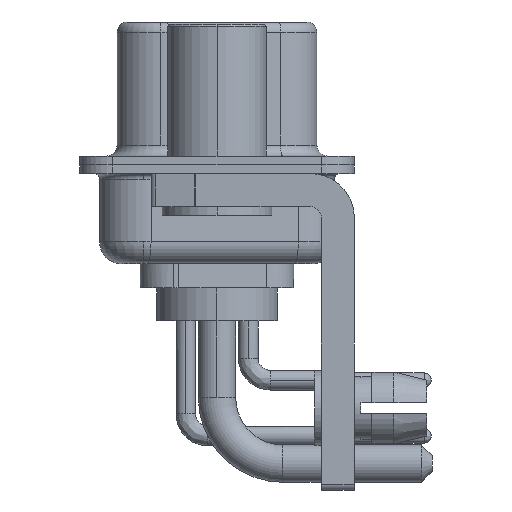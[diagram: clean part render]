
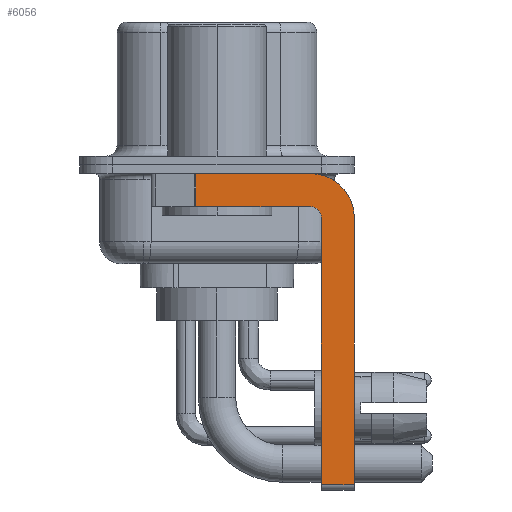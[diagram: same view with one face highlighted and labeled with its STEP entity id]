
A CAD part, left-side view. The second image highlights one B-rep face of the part: STEP entity #6056.
In plain terms, the highlighted planar face has unit normal (-1, 0, 0).
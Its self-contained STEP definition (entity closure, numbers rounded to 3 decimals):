
#176 = DIRECTION ( 'NONE',  ( 0., 0., -1. ) ) ;
#267 = CARTESIAN_POINT ( 'NONE',  ( -2.9, -4.75, -14.55 ) ) ;
#996 = DIRECTION ( 'NONE',  ( 0., 0., -1. ) ) ;
#1007 = AXIS2_PLACEMENT_3D ( 'NONE', #15987, #13909, #996 ) ;
#1122 = CARTESIAN_POINT ( 'NONE',  ( -2.9, -4.25, -2.4 ) ) ;
#1993 = VECTOR ( 'NONE', #10875, 1000. ) ;
#2012 = CARTESIAN_POINT ( 'NONE',  ( -2.9, -6.25, -14.55 ) ) ;
#2116 = ORIENTED_EDGE ( 'NONE', *, *, #15926, .F. ) ;
#2143 = CARTESIAN_POINT ( 'NONE',  ( -2.9, -4.75, -2.4 ) ) ;
#2294 = LINE ( 'NONE', #19380, #18590 ) ;
#2717 = CARTESIAN_POINT ( 'NONE',  ( -2.9, 0.978, -0.4 ) ) ;
#3073 = LINE ( 'NONE', #21999, #12347 ) ;
#3507 = CIRCLE ( 'NONE', #4383, 0.5 ) ;
#3719 = ORIENTED_EDGE ( 'NONE', *, *, #20674, .F. ) ;
#4383 = AXIS2_PLACEMENT_3D ( 'NONE', #13957, #26971, #12120 ) ;
#5748 = LINE ( 'NONE', #22566, #7154 ) ;
#6056 = ADVANCED_FACE ( 'NONE', ( #15854 ), #16405, .F. ) ;
#6746 = ORIENTED_EDGE ( 'NONE', *, *, #23729, .T. ) ;
#7154 = VECTOR ( 'NONE', #20450, 1000. ) ;
#7297 = ORIENTED_EDGE ( 'NONE', *, *, #23754, .F. ) ;
#7559 = EDGE_LOOP ( 'NONE', ( #9603, #21569, #16159, #3719, #18024, #6746, #2116, #7297 ) ) ;
#7631 = VERTEX_POINT ( 'NONE', #267 ) ;
#7816 = CARTESIAN_POINT ( 'NONE',  ( -2.9, -6.25, -2.4 ) ) ;
#7880 = VECTOR ( 'NONE', #22102, 1000. ) ;
#9040 = EDGE_CURVE ( 'NONE', #24967, #27465, #3073, .T. ) ;
#9541 = EDGE_CURVE ( 'NONE', #7631, #20826, #26171, .T. ) ;
#9603 = ORIENTED_EDGE ( 'NONE', *, *, #12255, .F. ) ;
#10739 = AXIS2_PLACEMENT_3D ( 'NONE', #1122, #24668, #16679 ) ;
#10875 = DIRECTION ( 'NONE',  ( 0., 1., 0. ) ) ;
#12120 = DIRECTION ( 'NONE',  ( 0., 0., 1. ) ) ;
#12238 = LINE ( 'NONE', #16596, #22991 ) ;
#12255 = EDGE_CURVE ( 'NONE', #24967, #17781, #12238, .T. ) ;
#12347 = VECTOR ( 'NONE', #13314, 1000. ) ;
#13314 = DIRECTION ( 'NONE',  ( 0., 0., -1. ) ) ;
#13909 = DIRECTION ( 'NONE',  ( 1., 0., 0. ) ) ;
#13957 = CARTESIAN_POINT ( 'NONE',  ( -2.9, -4.25, -2.4 ) ) ;
#14357 = VERTEX_POINT ( 'NONE', #15421 ) ;
#14451 = VERTEX_POINT ( 'NONE', #2012 ) ;
#15325 = EDGE_CURVE ( 'NONE', #14357, #27465, #24029, .T. ) ;
#15421 = CARTESIAN_POINT ( 'NONE',  ( -2.9, -4.25, -1.9 ) ) ;
#15480 = CARTESIAN_POINT ( 'NONE',  ( -2.9, 0.978, -1.9 ) ) ;
#15854 = FACE_OUTER_BOUND ( 'NONE', #7559, .T. ) ;
#15926 = EDGE_CURVE ( 'NONE', #22354, #14451, #2294, .T. ) ;
#15987 = CARTESIAN_POINT ( 'NONE',  ( -2.9, -4.25, -2.4 ) ) ;
#16159 = ORIENTED_EDGE ( 'NONE', *, *, #15325, .F. ) ;
#16405 = PLANE ( 'NONE',  #1007 ) ;
#16596 = CARTESIAN_POINT ( 'NONE',  ( -2.9, 3., -0.4 ) ) ;
#16679 = DIRECTION ( 'NONE',  ( 0., 0., -1. ) ) ;
#17763 = CARTESIAN_POINT ( 'NONE',  ( -2.9, -4.75, -14.8 ) ) ;
#17781 = VERTEX_POINT ( 'NONE', #19537 ) ;
#18024 = ORIENTED_EDGE ( 'NONE', *, *, #9541, .F. ) ;
#18590 = VECTOR ( 'NONE', #176, 1000. ) ;
#19380 = CARTESIAN_POINT ( 'NONE',  ( -2.9, -6.25, -2.4 ) ) ;
#19537 = CARTESIAN_POINT ( 'NONE',  ( -2.9, -4.25, -0.4 ) ) ;
#20450 = DIRECTION ( 'NONE',  ( 0., -1., 0. ) ) ;
#20674 = EDGE_CURVE ( 'NONE', #20826, #14357, #3507, .T. ) ;
#20826 = VERTEX_POINT ( 'NONE', #2143 ) ;
#21569 = ORIENTED_EDGE ( 'NONE', *, *, #9040, .T. ) ;
#21999 = CARTESIAN_POINT ( 'NONE',  ( -2.9, 0.978, -1.9 ) ) ;
#22102 = DIRECTION ( 'NONE',  ( 0., 0., 1. ) ) ;
#22354 = VERTEX_POINT ( 'NONE', #7816 ) ;
#22566 = CARTESIAN_POINT ( 'NONE',  ( -2.9, -4.25, -14.55 ) ) ;
#22821 = CIRCLE ( 'NONE', #10739, 2. ) ;
#22991 = VECTOR ( 'NONE', #25269, 1000. ) ;
#23614 = CARTESIAN_POINT ( 'NONE',  ( -2.9, -4.25, -1.9 ) ) ;
#23729 = EDGE_CURVE ( 'NONE', #7631, #14451, #5748, .T. ) ;
#23754 = EDGE_CURVE ( 'NONE', #17781, #22354, #22821, .T. ) ;
#24029 = LINE ( 'NONE', #23614, #1993 ) ;
#24668 = DIRECTION ( 'NONE',  ( 1., 0., 0. ) ) ;
#24967 = VERTEX_POINT ( 'NONE', #2717 ) ;
#25269 = DIRECTION ( 'NONE',  ( 0., -1., 0. ) ) ;
#26171 = LINE ( 'NONE', #17763, #7880 ) ;
#26971 = DIRECTION ( 'NONE',  ( -1., 0., 0. ) ) ;
#27465 = VERTEX_POINT ( 'NONE', #15480 ) ;
